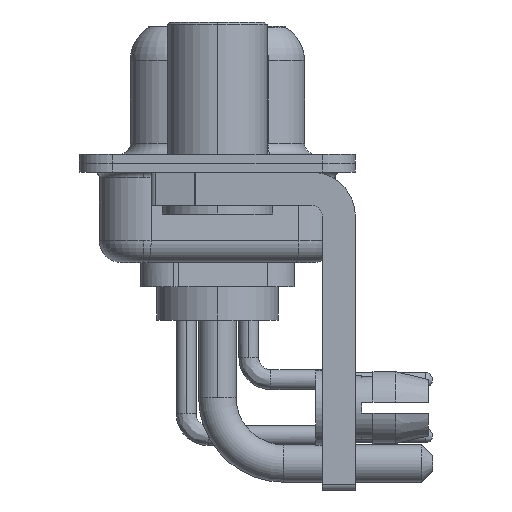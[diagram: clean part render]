
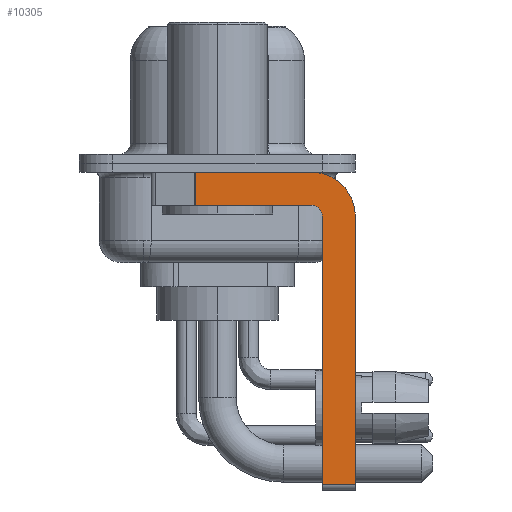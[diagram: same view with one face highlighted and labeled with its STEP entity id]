
A CAD part, left-side view. The second image highlights one B-rep face of the part: STEP entity #10305.
In plain terms, the highlighted planar face has unit normal (-1, 0, 0).
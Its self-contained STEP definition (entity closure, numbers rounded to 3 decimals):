
#335 = EDGE_CURVE ( 'NONE', #507, #26069, #9095, .T. ) ;
#376 = EDGE_LOOP ( 'NONE', ( #11834, #16207, #10379, #26089, #10234, #19510, #10742, #5108 ) ) ;
#507 = VERTEX_POINT ( 'NONE', #951 ) ;
#588 = VERTEX_POINT ( 'NONE', #9669 ) ;
#635 = AXIS2_PLACEMENT_3D ( 'NONE', #24759, #16561, #6534 ) ;
#951 = CARTESIAN_POINT ( 'NONE',  ( -2.9, -4.75, -2.4 ) ) ;
#1113 = EDGE_CURVE ( 'NONE', #588, #21385, #22777, .T. ) ;
#1115 = LINE ( 'NONE', #21098, #15823 ) ;
#3897 = VECTOR ( 'NONE', #11274, 1000. ) ;
#5108 = ORIENTED_EDGE ( 'NONE', *, *, #11463, .F. ) ;
#5851 = LINE ( 'NONE', #21960, #3897 ) ;
#6440 = FACE_OUTER_BOUND ( 'NONE', #376, .T. ) ;
#6534 = DIRECTION ( 'NONE',  ( 0., 0., 1. ) ) ;
#7283 = DIRECTION ( 'NONE',  ( 0., -1., 0. ) ) ;
#7379 = AXIS2_PLACEMENT_3D ( 'NONE', #13357, #21295, #21421 ) ;
#8829 = VERTEX_POINT ( 'NONE', #10303 ) ;
#9095 = CIRCLE ( 'NONE', #635, 0.5 ) ;
#9271 = CARTESIAN_POINT ( 'NONE',  ( -2.9, -4.25, -14.55 ) ) ;
#9669 = CARTESIAN_POINT ( 'NONE',  ( -2.9, 0.978, -0.4 ) ) ;
#10234 = ORIENTED_EDGE ( 'NONE', *, *, #18342, .F. ) ;
#10303 = CARTESIAN_POINT ( 'NONE',  ( -2.9, -6.25, -14.55 ) ) ;
#10305 = ADVANCED_FACE ( 'NONE', ( #6440 ), #24789, .F. ) ;
#10321 = EDGE_CURVE ( 'NONE', #26069, #21385, #1115, .T. ) ;
#10379 = ORIENTED_EDGE ( 'NONE', *, *, #10321, .F. ) ;
#10742 = ORIENTED_EDGE ( 'NONE', *, *, #19656, .F. ) ;
#10800 = CARTESIAN_POINT ( 'NONE',  ( -2.9, -6.25, -2.4 ) ) ;
#10926 = CARTESIAN_POINT ( 'NONE',  ( -2.9, -4.25, -2.4 ) ) ;
#11183 = DIRECTION ( 'NONE',  ( 0., 1., 0. ) ) ;
#11274 = DIRECTION ( 'NONE',  ( 0., -1., 0. ) ) ;
#11463 = EDGE_CURVE ( 'NONE', #18707, #20171, #13305, .T. ) ;
#11834 = ORIENTED_EDGE ( 'NONE', *, *, #16100, .F. ) ;
#12106 = VERTEX_POINT ( 'NONE', #14075 ) ;
#12323 = LINE ( 'NONE', #20380, #24191 ) ;
#13291 = VECTOR ( 'NONE', #24927, 1000. ) ;
#13305 = CIRCLE ( 'NONE', #7379, 2. ) ;
#13357 = CARTESIAN_POINT ( 'NONE',  ( -2.9, -4.25, -2.4 ) ) ;
#14075 = CARTESIAN_POINT ( 'NONE',  ( -2.9, -4.75, -14.55 ) ) ;
#14559 = AXIS2_PLACEMENT_3D ( 'NONE', #10926, #20580, #24923 ) ;
#14944 = CARTESIAN_POINT ( 'NONE',  ( -2.9, -6.25, -2.4 ) ) ;
#15328 = LINE ( 'NONE', #9271, #20916 ) ;
#15823 = VECTOR ( 'NONE', #11183, 1000. ) ;
#16100 = EDGE_CURVE ( 'NONE', #588, #18707, #5851, .T. ) ;
#16207 = ORIENTED_EDGE ( 'NONE', *, *, #1113, .T. ) ;
#16561 = DIRECTION ( 'NONE',  ( -1., 0., 0. ) ) ;
#16603 = LINE ( 'NONE', #10800, #13291 ) ;
#18303 = CARTESIAN_POINT ( 'NONE',  ( -2.9, 0.978, -1.9 ) ) ;
#18342 = EDGE_CURVE ( 'NONE', #12106, #507, #12323, .T. ) ;
#18388 = DIRECTION ( 'NONE',  ( 0., 0., 1. ) ) ;
#18707 = VERTEX_POINT ( 'NONE', #22337 ) ;
#19510 = ORIENTED_EDGE ( 'NONE', *, *, #20256, .T. ) ;
#19656 = EDGE_CURVE ( 'NONE', #20171, #8829, #16603, .T. ) ;
#19897 = DIRECTION ( 'NONE',  ( 0., 0., -1. ) ) ;
#20161 = CARTESIAN_POINT ( 'NONE',  ( -2.9, 0.978, -1.9 ) ) ;
#20171 = VERTEX_POINT ( 'NONE', #14944 ) ;
#20256 = EDGE_CURVE ( 'NONE', #12106, #8829, #15328, .T. ) ;
#20380 = CARTESIAN_POINT ( 'NONE',  ( -2.9, -4.75, -14.8 ) ) ;
#20580 = DIRECTION ( 'NONE',  ( 1., 0., 0. ) ) ;
#20916 = VECTOR ( 'NONE', #7283, 1000. ) ;
#21098 = CARTESIAN_POINT ( 'NONE',  ( -2.9, -4.25, -1.9 ) ) ;
#21295 = DIRECTION ( 'NONE',  ( 1., 0., 0. ) ) ;
#21385 = VERTEX_POINT ( 'NONE', #18303 ) ;
#21421 = DIRECTION ( 'NONE',  ( 0., 0., -1. ) ) ;
#21960 = CARTESIAN_POINT ( 'NONE',  ( -2.9, 3., -0.4 ) ) ;
#22337 = CARTESIAN_POINT ( 'NONE',  ( -2.9, -4.25, -0.4 ) ) ;
#22417 = VECTOR ( 'NONE', #19897, 1000. ) ;
#22777 = LINE ( 'NONE', #20161, #22417 ) ;
#23540 = CARTESIAN_POINT ( 'NONE',  ( -2.9, -4.25, -1.9 ) ) ;
#24191 = VECTOR ( 'NONE', #18388, 1000. ) ;
#24759 = CARTESIAN_POINT ( 'NONE',  ( -2.9, -4.25, -2.4 ) ) ;
#24789 = PLANE ( 'NONE',  #14559 ) ;
#24923 = DIRECTION ( 'NONE',  ( 0., 0., -1. ) ) ;
#24927 = DIRECTION ( 'NONE',  ( 0., 0., -1. ) ) ;
#26069 = VERTEX_POINT ( 'NONE', #23540 ) ;
#26089 = ORIENTED_EDGE ( 'NONE', *, *, #335, .F. ) ;
